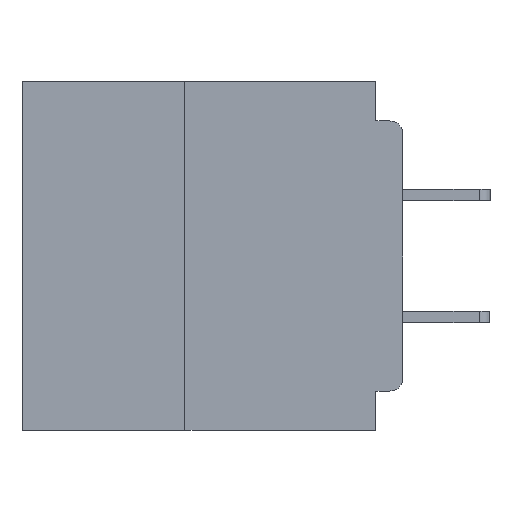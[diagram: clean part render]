
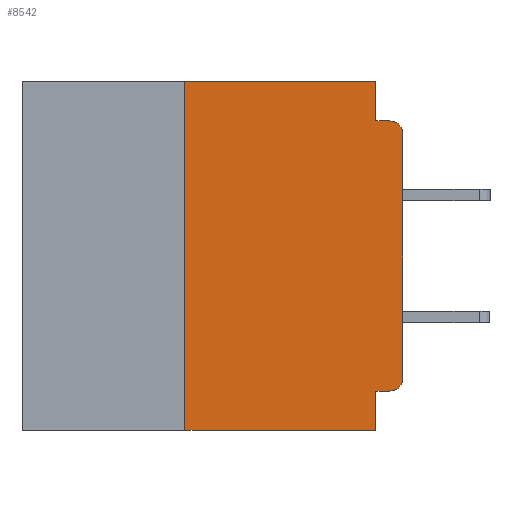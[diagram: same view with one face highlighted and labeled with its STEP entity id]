
A CAD part, left-side view. The second image highlights one B-rep face of the part: STEP entity #8542.
In plain terms, the highlighted planar face has unit normal (-1, 0, 0).
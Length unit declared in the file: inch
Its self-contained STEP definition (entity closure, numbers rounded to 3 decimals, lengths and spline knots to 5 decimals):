
#1297 = VECTOR ( 'NONE', #39677, 39.37008 ) ;
#1366 = ORIENTED_EDGE ( 'NONE', *, *, #47865, .F. ) ;
#2738 = DIRECTION ( 'NONE',  ( 0., 0., 1. ) ) ;
#3939 = CARTESIAN_POINT ( 'NONE',  ( 0., 0.015, -0.045 ) ) ;
#4986 = CARTESIAN_POINT ( 'NONE',  ( 0., 0.031, -0.4 ) ) ;
#5037 = LINE ( 'NONE', #33568, #38267 ) ;
#5190 = VECTOR ( 'NONE', #32601, 39.37008 ) ;
#5617 = PLANE ( 'NONE',  #50857 ) ;
#6740 = VERTEX_POINT ( 'NONE', #29794 ) ;
#7455 = EDGE_CURVE ( 'NONE', #7867, #33999, #24546, .T. ) ;
#7525 = VECTOR ( 'NONE', #2738, 39.37008 ) ;
#7867 = VERTEX_POINT ( 'NONE', #27149 ) ;
#8542 = ADVANCED_FACE ( 'NONE', ( #46158 ), #5617, .F. ) ;
#8983 = ORIENTED_EDGE ( 'NONE', *, *, #53749, .F. ) ;
#10343 = CARTESIAN_POINT ( 'NONE',  ( 0., 0.015, -0.06 ) ) ;
#10362 = DIRECTION ( 'NONE',  ( 0., 0., -1. ) ) ;
#11448 = CARTESIAN_POINT ( 'NONE',  ( 0., 0.031, 0. ) ) ;
#11651 = ORIENTED_EDGE ( 'NONE', *, *, #45715, .T. ) ;
#12494 = VECTOR ( 'NONE', #20562, 39.37008 ) ;
#12764 = CARTESIAN_POINT ( 'NONE',  ( 0., 0.437, 0. ) ) ;
#13700 = DIRECTION ( 'NONE',  ( 0., 0., -1. ) ) ;
#14311 = CARTESIAN_POINT ( 'NONE',  ( 0., 0.25, 0. ) ) ;
#14489 = VERTEX_POINT ( 'NONE', #51650 ) ;
#14672 = DIRECTION ( 'NONE',  ( 0., 0., -1. ) ) ;
#16188 = CARTESIAN_POINT ( 'NONE',  ( 0., 0., -0.045 ) ) ;
#16390 = ORIENTED_EDGE ( 'NONE', *, *, #29500, .T. ) ;
#17041 = VERTEX_POINT ( 'NONE', #30074 ) ;
#18490 = EDGE_CURVE ( 'NONE', #6740, #14489, #25211, .T. ) ;
#18892 = CARTESIAN_POINT ( 'NONE',  ( 0., 0.015, -0.34 ) ) ;
#20214 = VERTEX_POINT ( 'NONE', #14311 ) ;
#20562 = DIRECTION ( 'NONE',  ( 0., -1., 0. ) ) ;
#20983 = CARTESIAN_POINT ( 'NONE',  ( 0., 0.031, -0.045 ) ) ;
#21074 = ORIENTED_EDGE ( 'NONE', *, *, #18490, .T. ) ;
#21781 = ORIENTED_EDGE ( 'NONE', *, *, #48945, .T. ) ;
#22499 = ORIENTED_EDGE ( 'NONE', *, *, #53078, .F. ) ;
#22792 = EDGE_CURVE ( 'NONE', #20214, #7867, #47042, .T. ) ;
#23163 = VECTOR ( 'NONE', #50259, 39.37008 ) ;
#23267 = DIRECTION ( 'NONE',  ( 0., 0., -1. ) ) ;
#24066 = CARTESIAN_POINT ( 'NONE',  ( 0., 0., 0. ) ) ;
#24383 = CARTESIAN_POINT ( 'NONE',  ( 0., 0.25, -0.4 ) ) ;
#24546 = LINE ( 'NONE', #11448, #23163 ) ;
#25065 = DIRECTION ( 'NONE',  ( 0., -1., 0. ) ) ;
#25211 = CIRCLE ( 'NONE', #36276, 0.015 ) ;
#25420 = EDGE_CURVE ( 'NONE', #6740, #48404, #44753, .T. ) ;
#27149 = CARTESIAN_POINT ( 'NONE',  ( 0., 0.031, 0. ) ) ;
#29500 = EDGE_CURVE ( 'NONE', #29599, #55366, #5037, .T. ) ;
#29599 = VERTEX_POINT ( 'NONE', #43218 ) ;
#29794 = CARTESIAN_POINT ( 'NONE',  ( 0., 0.015, -0.355 ) ) ;
#30074 = CARTESIAN_POINT ( 'NONE',  ( 0., 0., -0.06 ) ) ;
#31158 = LINE ( 'NONE', #4986, #41292 ) ;
#31962 = CARTESIAN_POINT ( 'NONE',  ( 0., 0.437, 0. ) ) ;
#32601 = DIRECTION ( 'NONE',  ( 0., 0., 1. ) ) ;
#32646 = CARTESIAN_POINT ( 'NONE',  ( 0., 0.031, -0.355 ) ) ;
#33568 = CARTESIAN_POINT ( 'NONE',  ( 0., 0.437, -0.4 ) ) ;
#33999 = VERTEX_POINT ( 'NONE', #20983 ) ;
#35460 = LINE ( 'NONE', #16188, #12494 ) ;
#35471 = VECTOR ( 'NONE', #47381, 39.37008 ) ;
#35707 = AXIS2_PLACEMENT_3D ( 'NONE', #10343, #40615, #14672 ) ;
#36256 = DIRECTION ( 'NONE',  ( 1., 0., 0. ) ) ;
#36276 = AXIS2_PLACEMENT_3D ( 'NONE', #18892, #49196, #23267 ) ;
#38267 = VECTOR ( 'NONE', #25065, 39.37008 ) ;
#39677 = DIRECTION ( 'NONE',  ( 0., 1., 0. ) ) ;
#40615 = DIRECTION ( 'NONE',  ( -1., 0., 0. ) ) ;
#41106 = LINE ( 'NONE', #24066, #5190 ) ;
#41292 = VECTOR ( 'NONE', #13700, 39.37008 ) ;
#42764 = ORIENTED_EDGE ( 'NONE', *, *, #25420, .F. ) ;
#42926 = CARTESIAN_POINT ( 'NONE',  ( 0., 0.031, -0.4 ) ) ;
#43213 = CIRCLE ( 'NONE', #35707, 0.015 ) ;
#43218 = CARTESIAN_POINT ( 'NONE',  ( 0., 0.25, -0.4 ) ) ;
#44178 = ORIENTED_EDGE ( 'NONE', *, *, #22792, .F. ) ;
#44753 = LINE ( 'NONE', #52773, #1297 ) ;
#45715 = EDGE_CURVE ( 'NONE', #17041, #52613, #43213, .T. ) ;
#46158 = FACE_OUTER_BOUND ( 'NONE', #52963, .T. ) ;
#47042 = LINE ( 'NONE', #12764, #35471 ) ;
#47381 = DIRECTION ( 'NONE',  ( 0., -1., 0. ) ) ;
#47865 = EDGE_CURVE ( 'NONE', #33999, #52613, #35460, .T. ) ;
#48404 = VERTEX_POINT ( 'NONE', #32646 ) ;
#48945 = EDGE_CURVE ( 'NONE', #14489, #17041, #41106, .T. ) ;
#49196 = DIRECTION ( 'NONE',  ( -1., 0., 0. ) ) ;
#50259 = DIRECTION ( 'NONE',  ( 0., 0., -1. ) ) ;
#50857 = AXIS2_PLACEMENT_3D ( 'NONE', #31962, #36256, #10362 ) ;
#51630 = ORIENTED_EDGE ( 'NONE', *, *, #7455, .F. ) ;
#51650 = CARTESIAN_POINT ( 'NONE',  ( 0., 0., -0.34 ) ) ;
#52613 = VERTEX_POINT ( 'NONE', #3939 ) ;
#52773 = CARTESIAN_POINT ( 'NONE',  ( 0., 0., -0.355 ) ) ;
#52963 = EDGE_LOOP ( 'NONE', ( #21781, #11651, #1366, #51630, #44178, #22499, #16390, #8983, #42764, #21074 ) ) ;
#53078 = EDGE_CURVE ( 'NONE', #29599, #20214, #53572, .T. ) ;
#53572 = LINE ( 'NONE', #24383, #7525 ) ;
#53749 = EDGE_CURVE ( 'NONE', #48404, #55366, #31158, .T. ) ;
#55366 = VERTEX_POINT ( 'NONE', #42926 ) ;
